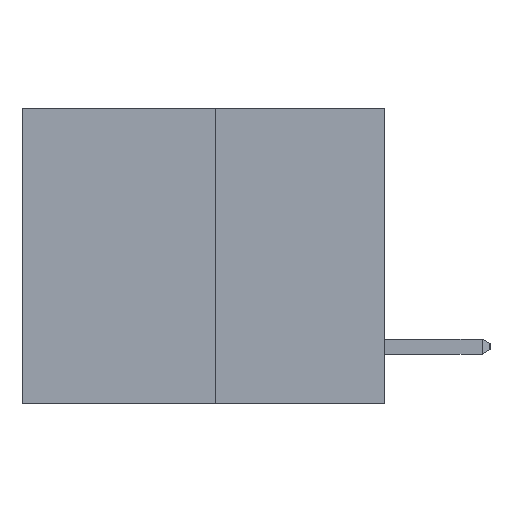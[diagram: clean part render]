
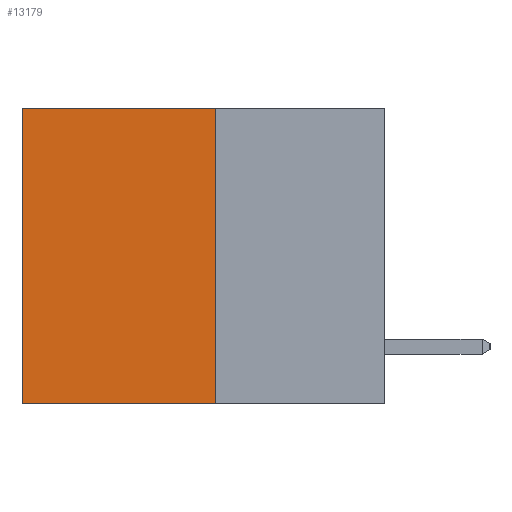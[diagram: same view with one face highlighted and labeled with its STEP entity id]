
A CAD part, left-side view. The second image highlights one B-rep face of the part: STEP entity #13179.
In plain terms, the highlighted planar face has unit normal (-1, 0, 0).
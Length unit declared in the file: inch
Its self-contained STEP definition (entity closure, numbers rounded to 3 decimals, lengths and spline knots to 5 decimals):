
#193 = EDGE_CURVE ( 'NONE', #6632, #19524, #1463, .T. ) ;
#684 = VECTOR ( 'NONE', #6672, 39.37008 ) ;
#809 = AXIS2_PLACEMENT_3D ( 'NONE', #15585, #20388, #10749 ) ;
#1340 = ORIENTED_EDGE ( 'NONE', *, *, #193, .F. ) ;
#1463 = LINE ( 'NONE', #11639, #4926 ) ;
#1804 = VERTEX_POINT ( 'NONE', #11034 ) ;
#1819 = CARTESIAN_POINT ( 'NONE',  ( 0.3165, 0.28, -0.49 ) ) ;
#3174 = LINE ( 'NONE', #17678, #684 ) ;
#3737 = CARTESIAN_POINT ( 'NONE',  ( 0.3165, 0.28, -0.49 ) ) ;
#4117 = LINE ( 'NONE', #1819, #10975 ) ;
#4766 = VERTEX_POINT ( 'NONE', #17969 ) ;
#4926 = VECTOR ( 'NONE', #5295, 39.37008 ) ;
#5295 = DIRECTION ( 'NONE',  ( 0., 0., -1. ) ) ;
#6621 = ORIENTED_EDGE ( 'NONE', *, *, #17597, .T. ) ;
#6632 = VERTEX_POINT ( 'NONE', #15839 ) ;
#6672 = DIRECTION ( 'NONE',  ( 0., 0., -1. ) ) ;
#6955 = EDGE_LOOP ( 'NONE', ( #17240, #7996, #1340, #6621 ) ) ;
#7811 = DIRECTION ( 'NONE',  ( 0., 1., 0. ) ) ;
#7996 = ORIENTED_EDGE ( 'NONE', *, *, #17630, .F. ) ;
#9006 = LINE ( 'NONE', #17168, #16656 ) ;
#9364 = PLANE ( 'NONE',  #809 ) ;
#10749 = DIRECTION ( 'NONE',  ( 0., 0., -1. ) ) ;
#10975 = VECTOR ( 'NONE', #12822, 39.37008 ) ;
#11034 = CARTESIAN_POINT ( 'NONE',  ( 0.3165, 0.6, -0.49 ) ) ;
#11639 = CARTESIAN_POINT ( 'NONE',  ( 0.3165, 0.28, -0.49 ) ) ;
#12822 = DIRECTION ( 'NONE',  ( 0., 1., 0. ) ) ;
#13179 = ADVANCED_FACE ( 'NONE', ( #15399 ), #9364, .F. ) ;
#15399 = FACE_OUTER_BOUND ( 'NONE', #6955, .T. ) ;
#15585 = CARTESIAN_POINT ( 'NONE',  ( 0.3165, 0.28, -0.49 ) ) ;
#15839 = CARTESIAN_POINT ( 'NONE',  ( 0.3165, 0.28, 0. ) ) ;
#15897 = EDGE_CURVE ( 'NONE', #4766, #1804, #3174, .T. ) ;
#16656 = VECTOR ( 'NONE', #7811, 39.37008 ) ;
#17168 = CARTESIAN_POINT ( 'NONE',  ( 0.3165, 0.28, 0. ) ) ;
#17240 = ORIENTED_EDGE ( 'NONE', *, *, #15897, .T. ) ;
#17597 = EDGE_CURVE ( 'NONE', #6632, #4766, #9006, .T. ) ;
#17630 = EDGE_CURVE ( 'NONE', #19524, #1804, #4117, .T. ) ;
#17678 = CARTESIAN_POINT ( 'NONE',  ( 0.3165, 0.6, -0.49 ) ) ;
#17969 = CARTESIAN_POINT ( 'NONE',  ( 0.3165, 0.6, 0. ) ) ;
#19524 = VERTEX_POINT ( 'NONE', #3737 ) ;
#20388 = DIRECTION ( 'NONE',  ( 1., 0., 0. ) ) ;
